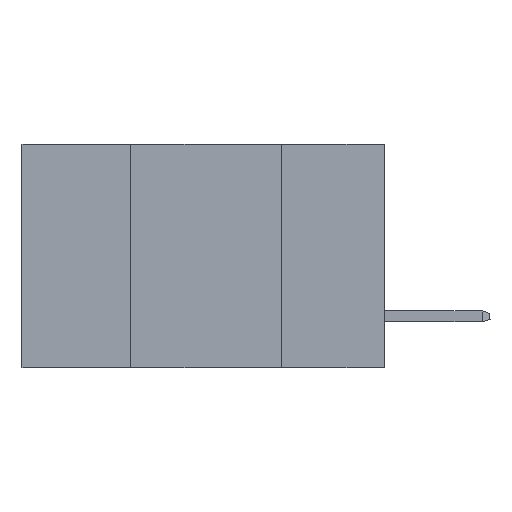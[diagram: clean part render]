
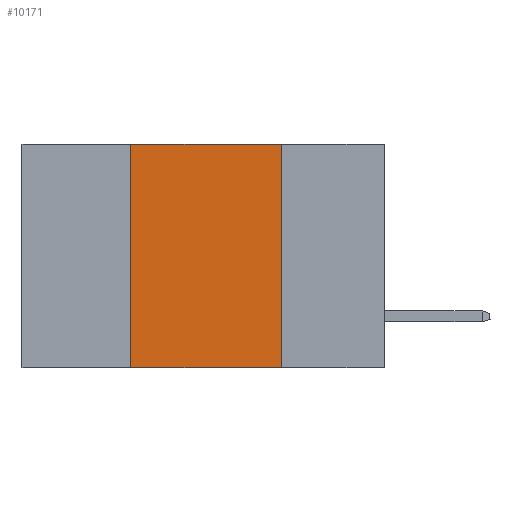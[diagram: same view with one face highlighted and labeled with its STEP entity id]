
A CAD part, left-side view. The second image highlights one B-rep face of the part: STEP entity #10171.
In plain terms, the highlighted planar face has unit normal (-1, 0, 0).
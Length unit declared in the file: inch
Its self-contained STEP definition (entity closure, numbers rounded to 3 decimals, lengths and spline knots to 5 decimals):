
#268 = LINE ( 'NONE', #6269, #2489 ) ;
#563 = DIRECTION ( 'NONE',  ( 0., 0., -1. ) ) ;
#1562 = ORIENTED_EDGE ( 'NONE', *, *, #9813, .F. ) ;
#1999 = VERTEX_POINT ( 'NONE', #3392 ) ;
#2489 = VECTOR ( 'NONE', #7389, 39.37008 ) ;
#2819 = DIRECTION ( 'NONE',  ( 1., 0., 0. ) ) ;
#2899 = AXIS2_PLACEMENT_3D ( 'NONE', #8410, #2819, #8367 ) ;
#3392 = CARTESIAN_POINT ( 'NONE',  ( 0., 0.42, -0.37 ) ) ;
#3571 = VERTEX_POINT ( 'NONE', #4058 ) ;
#3667 = ORIENTED_EDGE ( 'NONE', *, *, #6858, .F. ) ;
#4058 = CARTESIAN_POINT ( 'NONE',  ( 0., 0.17, 0. ) ) ;
#4343 = LINE ( 'NONE', #10350, #8815 ) ;
#4792 = CARTESIAN_POINT ( 'NONE',  ( 0., 0.17, 0. ) ) ;
#5118 = FACE_OUTER_BOUND ( 'NONE', #6507, .T. ) ;
#6269 = CARTESIAN_POINT ( 'NONE',  ( 0., 0.6, -0.37 ) ) ;
#6398 = LINE ( 'NONE', #7510, #10570 ) ;
#6507 = EDGE_LOOP ( 'NONE', ( #1562, #3667, #14021, #7491 ) ) ;
#6858 = EDGE_CURVE ( 'NONE', #7898, #3571, #6398, .T. ) ;
#7389 = DIRECTION ( 'NONE',  ( 0., -1., 0. ) ) ;
#7491 = ORIENTED_EDGE ( 'NONE', *, *, #12427, .T. ) ;
#7510 = CARTESIAN_POINT ( 'NONE',  ( 0., 0.6, 0. ) ) ;
#7898 = VERTEX_POINT ( 'NONE', #13103 ) ;
#7934 = EDGE_CURVE ( 'NONE', #1999, #7898, #4343, .T. ) ;
#8367 = DIRECTION ( 'NONE',  ( 0., 0., -1. ) ) ;
#8410 = CARTESIAN_POINT ( 'NONE',  ( 0., 0.6, 0. ) ) ;
#8815 = VECTOR ( 'NONE', #9273, 39.37008 ) ;
#9273 = DIRECTION ( 'NONE',  ( 0., 0., 1. ) ) ;
#9437 = VERTEX_POINT ( 'NONE', #10119 ) ;
#9686 = DIRECTION ( 'NONE',  ( 0., -1., 0. ) ) ;
#9813 = EDGE_CURVE ( 'NONE', #3571, #9437, #10469, .T. ) ;
#10119 = CARTESIAN_POINT ( 'NONE',  ( 0., 0.17, -0.37 ) ) ;
#10171 = ADVANCED_FACE ( 'NONE', ( #5118 ), #13897, .F. ) ;
#10350 = CARTESIAN_POINT ( 'NONE',  ( 0., 0.42, 0. ) ) ;
#10469 = LINE ( 'NONE', #4792, #12669 ) ;
#10570 = VECTOR ( 'NONE', #9686, 39.37008 ) ;
#12427 = EDGE_CURVE ( 'NONE', #1999, #9437, #268, .T. ) ;
#12669 = VECTOR ( 'NONE', #563, 39.37008 ) ;
#13103 = CARTESIAN_POINT ( 'NONE',  ( 0., 0.42, 0. ) ) ;
#13897 = PLANE ( 'NONE',  #2899 ) ;
#14021 = ORIENTED_EDGE ( 'NONE', *, *, #7934, .F. ) ;
